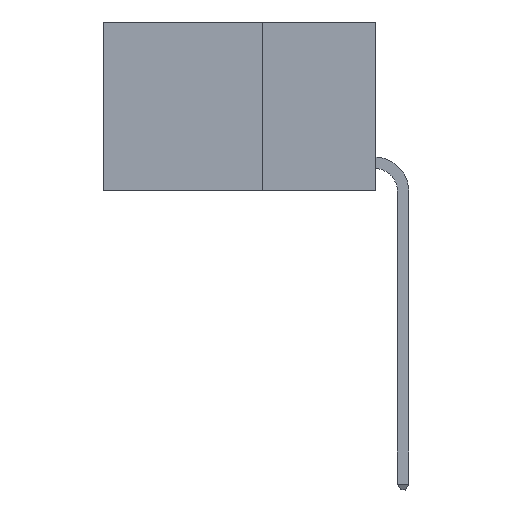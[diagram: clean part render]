
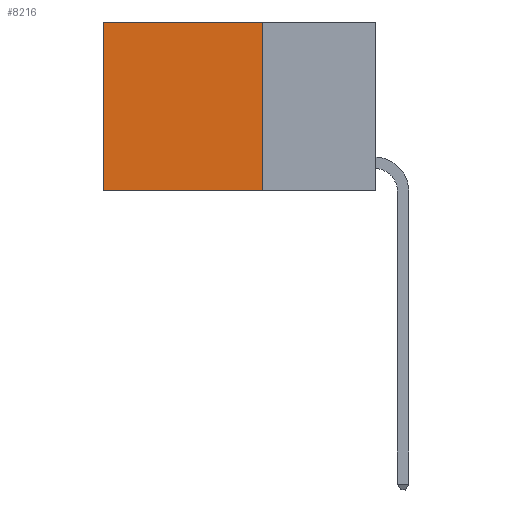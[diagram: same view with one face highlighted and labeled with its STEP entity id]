
A CAD part, left-side view. The second image highlights one B-rep face of the part: STEP entity #8216.
In plain terms, the highlighted planar face has unit normal (-1, 0, 0).
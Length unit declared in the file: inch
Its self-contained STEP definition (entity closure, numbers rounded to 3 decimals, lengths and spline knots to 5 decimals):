
#500 = CARTESIAN_POINT ( 'NONE',  ( 0.2625, 0.6, 0. ) ) ;
#1186 = VERTEX_POINT ( 'NONE', #16340 ) ;
#1247 = CARTESIAN_POINT ( 'NONE',  ( 0.2625, 0.25, -0.37 ) ) ;
#1302 = DIRECTION ( 'NONE',  ( 0., 1., 0. ) ) ;
#1744 = CARTESIAN_POINT ( 'NONE',  ( 0.2625, 0.6, -0.37 ) ) ;
#2491 = CARTESIAN_POINT ( 'NONE',  ( 0.2625, 0.25, 0. ) ) ;
#2693 = DIRECTION ( 'NONE',  ( 0., 0., -1. ) ) ;
#2745 = AXIS2_PLACEMENT_3D ( 'NONE', #2491, #12151, #3900 ) ;
#3251 = ORIENTED_EDGE ( 'NONE', *, *, #7700, .F. ) ;
#3655 = VERTEX_POINT ( 'NONE', #1744 ) ;
#3900 = DIRECTION ( 'NONE',  ( 0., 0., -1. ) ) ;
#4421 = VECTOR ( 'NONE', #16327, 39.37008 ) ;
#5276 = CARTESIAN_POINT ( 'NONE',  ( 0.2625, 0.25, 0. ) ) ;
#6809 = VECTOR ( 'NONE', #1302, 39.37008 ) ;
#7336 = VERTEX_POINT ( 'NONE', #15776 ) ;
#7425 = LINE ( 'NONE', #500, #11481 ) ;
#7700 = EDGE_CURVE ( 'NONE', #1186, #7336, #17561, .T. ) ;
#8054 = FACE_OUTER_BOUND ( 'NONE', #16984, .T. ) ;
#8098 = LINE ( 'NONE', #5276, #4421 ) ;
#8216 = ADVANCED_FACE ( 'NONE', ( #8054 ), #17659, .F. ) ;
#8710 = ORIENTED_EDGE ( 'NONE', *, *, #13704, .F. ) ;
#9561 = ORIENTED_EDGE ( 'NONE', *, *, #13631, .T. ) ;
#9893 = CARTESIAN_POINT ( 'NONE',  ( 0.2625, 0.6, 0. ) ) ;
#10159 = DIRECTION ( 'NONE',  ( 0., 0., -1. ) ) ;
#10264 = VERTEX_POINT ( 'NONE', #9893 ) ;
#11481 = VECTOR ( 'NONE', #10159, 39.37008 ) ;
#12151 = DIRECTION ( 'NONE',  ( 1., 0., 0. ) ) ;
#12935 = ORIENTED_EDGE ( 'NONE', *, *, #14368, .T. ) ;
#13463 = VECTOR ( 'NONE', #2693, 39.37008 ) ;
#13631 = EDGE_CURVE ( 'NONE', #1186, #10264, #8098, .T. ) ;
#13704 = EDGE_CURVE ( 'NONE', #7336, #3655, #14131, .T. ) ;
#14131 = LINE ( 'NONE', #1247, #6809 ) ;
#14368 = EDGE_CURVE ( 'NONE', #10264, #3655, #7425, .T. ) ;
#15106 = CARTESIAN_POINT ( 'NONE',  ( 0.2625, 0.25, 0. ) ) ;
#15776 = CARTESIAN_POINT ( 'NONE',  ( 0.2625, 0.25, -0.37 ) ) ;
#16327 = DIRECTION ( 'NONE',  ( 0., 1., 0. ) ) ;
#16340 = CARTESIAN_POINT ( 'NONE',  ( 0.2625, 0.25, 0. ) ) ;
#16984 = EDGE_LOOP ( 'NONE', ( #12935, #8710, #3251, #9561 ) ) ;
#17561 = LINE ( 'NONE', #15106, #13463 ) ;
#17659 = PLANE ( 'NONE',  #2745 ) ;
